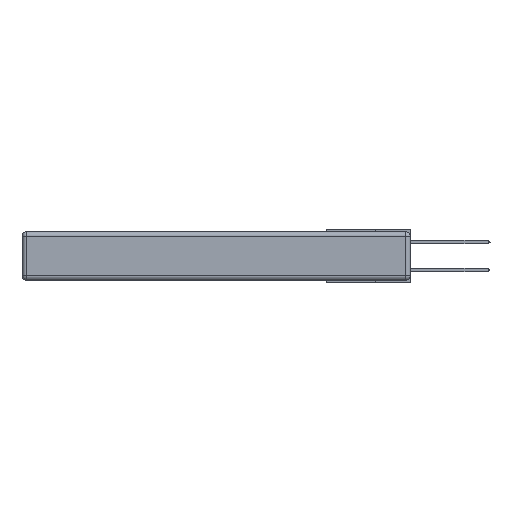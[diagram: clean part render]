
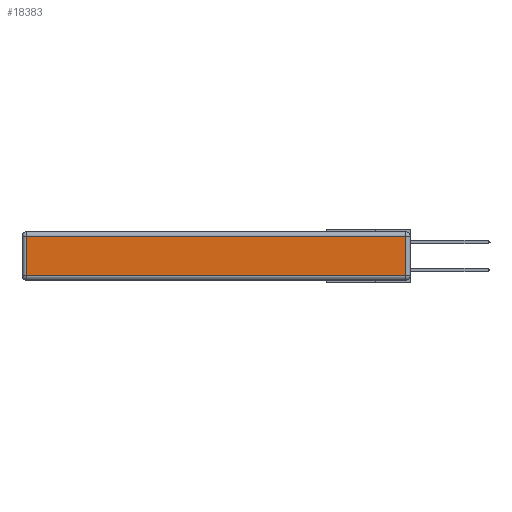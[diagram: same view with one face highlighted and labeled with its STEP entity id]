
A CAD part, left-side view. The second image highlights one B-rep face of the part: STEP entity #18383.
In plain terms, the highlighted planar face has unit normal (-1, 0, 0).
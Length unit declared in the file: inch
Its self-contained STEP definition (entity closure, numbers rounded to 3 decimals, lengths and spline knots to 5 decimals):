
#861 = VECTOR ( 'NONE', #23483, 39.37008 ) ;
#1747 = LINE ( 'NONE', #21961, #20466 ) ;
#2040 = AXIS2_PLACEMENT_3D ( 'NONE', #12915, #5251, #18747 ) ;
#2401 = EDGE_CURVE ( 'NONE', #11376, #11556, #6221, .T. ) ;
#4008 = CARTESIAN_POINT ( 'NONE',  ( 0., 0.03, -0.343 ) ) ;
#4124 = ORIENTED_EDGE ( 'NONE', *, *, #17230, .T. ) ;
#4453 = CARTESIAN_POINT ( 'NONE',  ( 0., 2.72, -0.343 ) ) ;
#5251 = DIRECTION ( 'NONE',  ( -1., 0., 0. ) ) ;
#5974 = LINE ( 'NONE', #4008, #861 ) ;
#6221 = LINE ( 'NONE', #4453, #15905 ) ;
#6639 = EDGE_CURVE ( 'NONE', #11556, #14152, #23586, .T. ) ;
#7421 = DIRECTION ( 'NONE',  ( 0., -1., 0. ) ) ;
#7495 = CARTESIAN_POINT ( 'NONE',  ( 0., 2.72, -0.03 ) ) ;
#11376 = VERTEX_POINT ( 'NONE', #7495 ) ;
#11556 = VERTEX_POINT ( 'NONE', #22750 ) ;
#12020 = CARTESIAN_POINT ( 'NONE',  ( 0., 0.03, -0.313 ) ) ;
#12189 = CARTESIAN_POINT ( 'NONE',  ( 0., 0.03, -0.03 ) ) ;
#12915 = CARTESIAN_POINT ( 'NONE',  ( 0., 0., -0.343 ) ) ;
#13537 = VECTOR ( 'NONE', #7421, 39.37008 ) ;
#14152 = VERTEX_POINT ( 'NONE', #12020 ) ;
#14306 = DIRECTION ( 'NONE',  ( 0., 0., -1. ) ) ;
#15905 = VECTOR ( 'NONE', #14306, 39.37008 ) ;
#16009 = ORIENTED_EDGE ( 'NONE', *, *, #6639, .T. ) ;
#16343 = DIRECTION ( 'NONE',  ( 0., 1., 0. ) ) ;
#17048 = EDGE_CURVE ( 'NONE', #23179, #11376, #1747, .T. ) ;
#17230 = EDGE_CURVE ( 'NONE', #14152, #23179, #5974, .T. ) ;
#17549 = EDGE_LOOP ( 'NONE', ( #16009, #4124, #18803, #19947 ) ) ;
#18383 = ADVANCED_FACE ( 'NONE', ( #21236 ), #24538, .T. ) ;
#18747 = DIRECTION ( 'NONE',  ( 0., 0., 1. ) ) ;
#18803 = ORIENTED_EDGE ( 'NONE', *, *, #17048, .T. ) ;
#19947 = ORIENTED_EDGE ( 'NONE', *, *, #2401, .T. ) ;
#20466 = VECTOR ( 'NONE', #16343, 39.37008 ) ;
#20590 = CARTESIAN_POINT ( 'NONE',  ( 0., 0., -0.313 ) ) ;
#21236 = FACE_OUTER_BOUND ( 'NONE', #17549, .T. ) ;
#21961 = CARTESIAN_POINT ( 'NONE',  ( 0., 2.75, -0.03 ) ) ;
#22750 = CARTESIAN_POINT ( 'NONE',  ( 0., 2.72, -0.313 ) ) ;
#23179 = VERTEX_POINT ( 'NONE', #12189 ) ;
#23483 = DIRECTION ( 'NONE',  ( 0., 0., 1. ) ) ;
#23586 = LINE ( 'NONE', #20590, #13537 ) ;
#24538 = PLANE ( 'NONE',  #2040 ) ;
